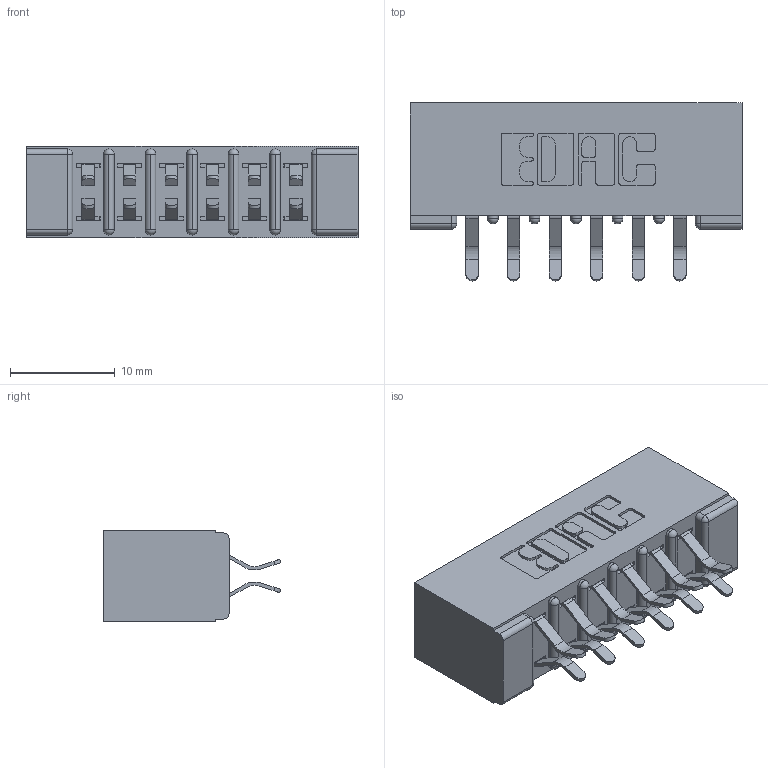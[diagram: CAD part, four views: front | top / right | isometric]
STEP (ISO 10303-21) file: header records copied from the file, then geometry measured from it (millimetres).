
FILE_DESCRIPTION (( 'STEP AP203' ), '1' );
FILE_NAME ('357-012-456-201.STEP', '2020-10-02T16:39:29', ( '' ), ( '' ), 'SwSTEP 2.0', 'SolidWorks 2020', '' );
FILE_SCHEMA (( 'CONFIG_CONTROL_DESIGN' ));
Length unit declared in the file: inch
Products named in the file (3): 307-290-001_556; 307 Part_No Mounting Lugs; 357-012-456-201
Assembly tree (13 placements, depth 2):
  357-012-456-201
    307 Part_No Mounting Lugs
    307-290-001_556  x12
Bounding box: 31.65 x 16.97 x 8.71 mm (x, y, z)
Volume: 2302.9 mm3; surface area: 3691.7 mm2
Topology: 13 solids, 13 shells, 717 faces, 2003 edges, 1298 vertices
Faces by surface type: plane 462, cylinder 241, sphere 14
Entity records: 9600 total; most frequent: CARTESIAN_POINT 1578, DIRECTION 1561, ORIENTED_EDGE 1558, EDGE_CURVE 779, LINE 583, VECTOR 583, VERTEX_POINT 506, AXIS2_PLACEMENT_3D 489
